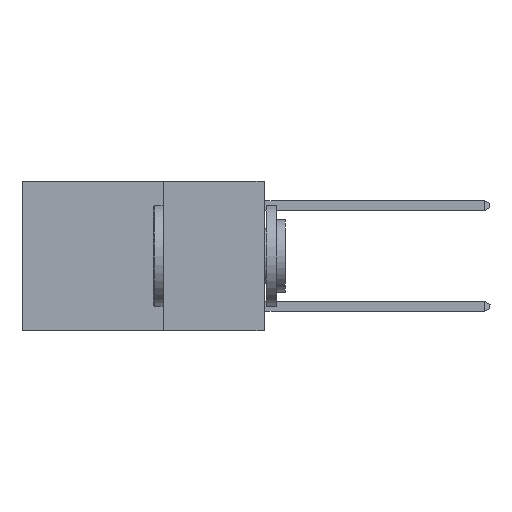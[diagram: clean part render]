
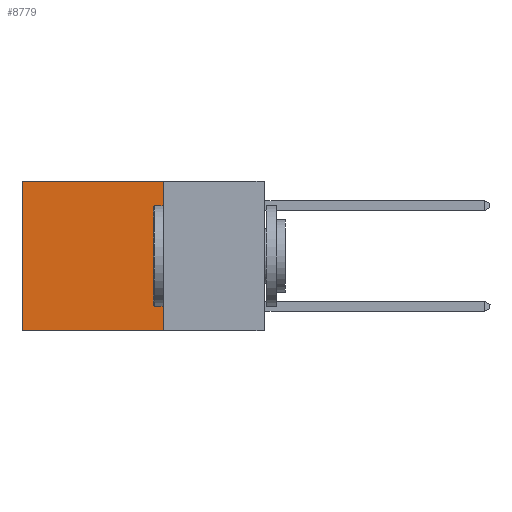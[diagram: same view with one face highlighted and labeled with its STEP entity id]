
A CAD part, left-side view. The second image highlights one B-rep face of the part: STEP entity #8779.
In plain terms, the highlighted planar face has unit normal (-1, 0, 0).
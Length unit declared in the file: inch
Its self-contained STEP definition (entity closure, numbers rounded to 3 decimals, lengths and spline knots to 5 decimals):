
#189 = CARTESIAN_POINT ( 'NONE',  ( 0.2625, 0.25, 0. ) ) ;
#336 = CARTESIAN_POINT ( 'NONE',  ( 0.2625, 0.25, 0. ) ) ;
#597 = LINE ( 'NONE', #6765, #6458 ) ;
#1076 = ORIENTED_EDGE ( 'NONE', *, *, #9589, .T. ) ;
#1135 = DIRECTION ( 'NONE',  ( 0., 1., 0. ) ) ;
#1868 = CARTESIAN_POINT ( 'NONE',  ( 0.2625, 0.25, 0. ) ) ;
#2476 = ORIENTED_EDGE ( 'NONE', *, *, #11495, .F. ) ;
#3009 = CARTESIAN_POINT ( 'NONE',  ( 0.2625, 0.6, -0.37 ) ) ;
#3065 = PLANE ( 'NONE',  #13550 ) ;
#3807 = DIRECTION ( 'NONE',  ( 0., 0., -1. ) ) ;
#4106 = EDGE_CURVE ( 'NONE', #9950, #4529, #6416, .T. ) ;
#4225 = DIRECTION ( 'NONE',  ( 1., 0., 0. ) ) ;
#4529 = VERTEX_POINT ( 'NONE', #14912 ) ;
#4609 = VECTOR ( 'NONE', #3807, 39.37008 ) ;
#4795 = VECTOR ( 'NONE', #1135, 39.37008 ) ;
#5324 = CARTESIAN_POINT ( 'NONE',  ( 0.2625, 0.25, -0.37 ) ) ;
#5407 = FACE_OUTER_BOUND ( 'NONE', #13692, .T. ) ;
#5424 = EDGE_CURVE ( 'NONE', #9950, #13650, #7668, .T. ) ;
#6416 = LINE ( 'NONE', #8116, #4795 ) ;
#6458 = VECTOR ( 'NONE', #12628, 39.37008 ) ;
#6765 = CARTESIAN_POINT ( 'NONE',  ( 0.2625, 0.6, 0. ) ) ;
#7668 = LINE ( 'NONE', #189, #4609 ) ;
#8116 = CARTESIAN_POINT ( 'NONE',  ( 0.2625, 0.25, 0. ) ) ;
#8415 = DIRECTION ( 'NONE',  ( 0., 1., 0. ) ) ;
#8779 = ADVANCED_FACE ( 'NONE', ( #5407 ), #3065, .F. ) ;
#8954 = VECTOR ( 'NONE', #8415, 39.37008 ) ;
#9589 = EDGE_CURVE ( 'NONE', #4529, #10746, #597, .T. ) ;
#9950 = VERTEX_POINT ( 'NONE', #336 ) ;
#10746 = VERTEX_POINT ( 'NONE', #3009 ) ;
#11000 = ORIENTED_EDGE ( 'NONE', *, *, #4106, .T. ) ;
#11495 = EDGE_CURVE ( 'NONE', #13650, #10746, #12091, .T. ) ;
#12091 = LINE ( 'NONE', #14237, #8954 ) ;
#12354 = DIRECTION ( 'NONE',  ( 0., 0., -1. ) ) ;
#12628 = DIRECTION ( 'NONE',  ( 0., 0., -1. ) ) ;
#12856 = ORIENTED_EDGE ( 'NONE', *, *, #5424, .F. ) ;
#13550 = AXIS2_PLACEMENT_3D ( 'NONE', #1868, #4225, #12354 ) ;
#13650 = VERTEX_POINT ( 'NONE', #5324 ) ;
#13692 = EDGE_LOOP ( 'NONE', ( #1076, #2476, #12856, #11000 ) ) ;
#14237 = CARTESIAN_POINT ( 'NONE',  ( 0.2625, 0.25, -0.37 ) ) ;
#14912 = CARTESIAN_POINT ( 'NONE',  ( 0.2625, 0.6, 0. ) ) ;
